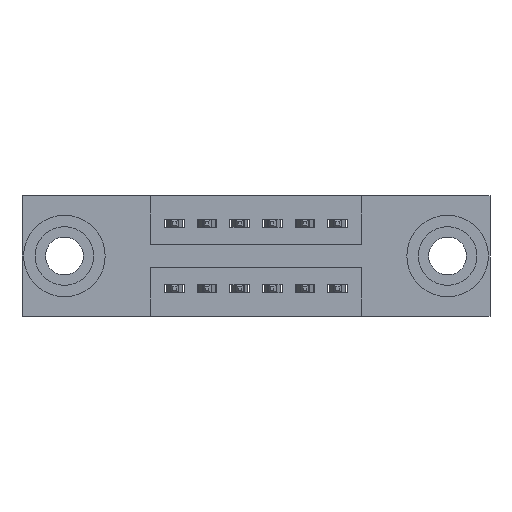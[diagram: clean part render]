
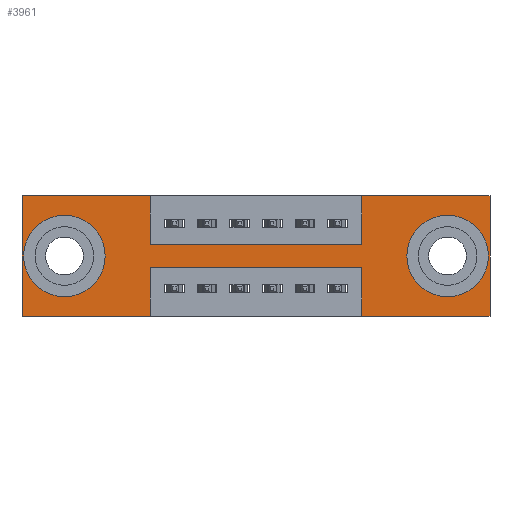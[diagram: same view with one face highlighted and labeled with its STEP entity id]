
A CAD part, front view. The second image highlights one B-rep face of the part: STEP entity #3961.
In plain terms, the highlighted planar face has unit normal (0, -1, 0).
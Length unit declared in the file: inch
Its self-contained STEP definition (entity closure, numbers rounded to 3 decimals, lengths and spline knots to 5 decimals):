
#34 = DIRECTION ( 'NONE',  ( 0., 0., -1. ) ) ;
#42 = VERTEX_POINT ( 'NONE', #1197 ) ;
#92 = CARTESIAN_POINT ( 'NONE',  ( 0., 0., -0.37 ) ) ;
#171 = DIRECTION ( 'NONE',  ( 1., 0., 0. ) ) ;
#291 = ORIENTED_EDGE ( 'NONE', *, *, #3632, .F. ) ;
#335 = AXIS2_PLACEMENT_3D ( 'NONE', #6196, #7779, #588 ) ;
#345 = CARTESIAN_POINT ( 'NONE',  ( 0.13, 0., -0.185 ) ) ;
#395 = ORIENTED_EDGE ( 'NONE', *, *, #940, .F. ) ;
#414 = VERTEX_POINT ( 'NONE', #714 ) ;
#434 = DIRECTION ( 'NONE',  ( 0., -1., 0. ) ) ;
#467 = CARTESIAN_POINT ( 'NONE',  ( 0., 0., 0. ) ) ;
#563 = EDGE_CURVE ( 'NONE', #6876, #4122, #4828, .T. ) ;
#571 = CARTESIAN_POINT ( 'NONE',  ( 1.0425, 0., 0. ) ) ;
#588 = DIRECTION ( 'NONE',  ( 0., 0., -1. ) ) ;
#666 = ORIENTED_EDGE ( 'NONE', *, *, #8290, .F. ) ;
#674 = VECTOR ( 'NONE', #724, 39.37008 ) ;
#714 = CARTESIAN_POINT ( 'NONE',  ( 0.3925, 0., -0.22 ) ) ;
#724 = DIRECTION ( 'NONE',  ( 1., 0., 0. ) ) ;
#737 = EDGE_CURVE ( 'NONE', #7230, #2003, #8035, .T. ) ;
#739 = CIRCLE ( 'NONE', #6644, 0.078 ) ;
#795 = ORIENTED_EDGE ( 'NONE', *, *, #1327, .F. ) ;
#940 = EDGE_CURVE ( 'NONE', #2744, #7206, #5294, .T. ) ;
#1187 = VECTOR ( 'NONE', #8932, 39.37008 ) ;
#1197 = CARTESIAN_POINT ( 'NONE',  ( 0.3925, 0., -0.15 ) ) ;
#1201 = VECTOR ( 'NONE', #8632, 39.37008 ) ;
#1287 = EDGE_CURVE ( 'NONE', #6546, #9096, #7022, .T. ) ;
#1300 = DIRECTION ( 'NONE',  ( 1., 0., 0. ) ) ;
#1327 = EDGE_CURVE ( 'NONE', #4214, #7230, #3807, .T. ) ;
#1444 = EDGE_CURVE ( 'NONE', #6327, #7670, #5656, .T. ) ;
#1595 = ORIENTED_EDGE ( 'NONE', *, *, #1444, .F. ) ;
#1898 = EDGE_CURVE ( 'NONE', #9096, #6546, #739, .T. ) ;
#1931 = LINE ( 'NONE', #2389, #1201 ) ;
#2003 = VERTEX_POINT ( 'NONE', #5486 ) ;
#2044 = CARTESIAN_POINT ( 'NONE',  ( 1.0425, 0., 0. ) ) ;
#2093 = EDGE_CURVE ( 'NONE', #8077, #414, #1931, .T. ) ;
#2120 = LINE ( 'NONE', #4509, #7315 ) ;
#2130 = VECTOR ( 'NONE', #1300, 39.37008 ) ;
#2210 = ORIENTED_EDGE ( 'NONE', *, *, #3200, .T. ) ;
#2382 = LINE ( 'NONE', #9507, #8199 ) ;
#2389 = CARTESIAN_POINT ( 'NONE',  ( 0.3925, 0., -0.22 ) ) ;
#2440 = EDGE_LOOP ( 'NONE', ( #5315, #8409 ) ) ;
#2575 = VECTOR ( 'NONE', #8770, 39.37008 ) ;
#2744 = VERTEX_POINT ( 'NONE', #4834 ) ;
#2754 = EDGE_LOOP ( 'NONE', ( #7285, #3383, #3017, #5675, #795, #291, #395, #4538, #8168, #666, #6199, #1595 ) ) ;
#2786 = PLANE ( 'NONE',  #6846 ) ;
#2809 = VECTOR ( 'NONE', #9680, 39.37008 ) ;
#2816 = VECTOR ( 'NONE', #171, 39.37008 ) ;
#2968 = CARTESIAN_POINT ( 'NONE',  ( 1.435, 0., -0.37 ) ) ;
#3017 = ORIENTED_EDGE ( 'NONE', *, *, #5569, .F. ) ;
#3023 = EDGE_CURVE ( 'NONE', #414, #6327, #8112, .T. ) ;
#3105 = DIRECTION ( 'NONE',  ( 0., 1., 0. ) ) ;
#3200 = EDGE_CURVE ( 'NONE', #4122, #6876, #6123, .T. ) ;
#3363 = CARTESIAN_POINT ( 'NONE',  ( 0.3925, 0., -0.37 ) ) ;
#3383 = ORIENTED_EDGE ( 'NONE', *, *, #2093, .F. ) ;
#3570 = DIRECTION ( 'NONE',  ( 0., 0., 1. ) ) ;
#3632 = EDGE_CURVE ( 'NONE', #7206, #4214, #7456, .T. ) ;
#3633 = FACE_BOUND ( 'NONE', #3957, .T. ) ;
#3665 = CARTESIAN_POINT ( 'NONE',  ( 1.0425, 0., -0.37 ) ) ;
#3807 = LINE ( 'NONE', #7151, #2575 ) ;
#3957 = EDGE_LOOP ( 'NONE', ( #7525, #2210 ) ) ;
#3961 = ADVANCED_FACE ( 'NONE', ( #3633, #7321, #5119 ), #2786, .T. ) ;
#4122 = VERTEX_POINT ( 'NONE', #8768 ) ;
#4139 = DIRECTION ( 'NONE',  ( 0., 1., 0. ) ) ;
#4182 = CARTESIAN_POINT ( 'NONE',  ( 0., 0., -0.37 ) ) ;
#4214 = VERTEX_POINT ( 'NONE', #7211 ) ;
#4333 = VECTOR ( 'NONE', #8064, 39.37008 ) ;
#4413 = VECTOR ( 'NONE', #5280, 39.37008 ) ;
#4509 = CARTESIAN_POINT ( 'NONE',  ( 0.3925, 0., 0. ) ) ;
#4538 = ORIENTED_EDGE ( 'NONE', *, *, #4627, .F. ) ;
#4627 = EDGE_CURVE ( 'NONE', #42, #2744, #4930, .T. ) ;
#4649 = AXIS2_PLACEMENT_3D ( 'NONE', #5413, #4139, #34 ) ;
#4743 = DIRECTION ( 'NONE',  ( 0., 0., 1. ) ) ;
#4828 = CIRCLE ( 'NONE', #4649, 0.078 ) ;
#4834 = CARTESIAN_POINT ( 'NONE',  ( 1.0425, 0., -0.15 ) ) ;
#4930 = LINE ( 'NONE', #8041, #2816 ) ;
#5119 = FACE_OUTER_BOUND ( 'NONE', #2754, .T. ) ;
#5280 = DIRECTION ( 'NONE',  ( 0., 0., 1. ) ) ;
#5294 = LINE ( 'NONE', #2044, #6050 ) ;
#5315 = ORIENTED_EDGE ( 'NONE', *, *, #1287, .T. ) ;
#5323 = CARTESIAN_POINT ( 'NONE',  ( 0.13, 0., -0.107 ) ) ;
#5381 = CARTESIAN_POINT ( 'NONE',  ( 0., 0., 0. ) ) ;
#5413 = CARTESIAN_POINT ( 'NONE',  ( 1.305, 0., -0.185 ) ) ;
#5486 = CARTESIAN_POINT ( 'NONE',  ( 1.0425, 0., -0.37 ) ) ;
#5569 = EDGE_CURVE ( 'NONE', #2003, #8077, #9389, .T. ) ;
#5656 = LINE ( 'NONE', #92, #2809 ) ;
#5675 = ORIENTED_EDGE ( 'NONE', *, *, #737, .F. ) ;
#5862 = CARTESIAN_POINT ( 'NONE',  ( 0., 0., 0. ) ) ;
#5942 = DIRECTION ( 'NONE',  ( 0., 0., -1. ) ) ;
#6004 = DIRECTION ( 'NONE',  ( 0., 0., 1. ) ) ;
#6050 = VECTOR ( 'NONE', #6004, 39.37008 ) ;
#6123 = CIRCLE ( 'NONE', #335, 0.078 ) ;
#6196 = CARTESIAN_POINT ( 'NONE',  ( 1.305, 0., -0.185 ) ) ;
#6199 = ORIENTED_EDGE ( 'NONE', *, *, #8209, .F. ) ;
#6327 = VERTEX_POINT ( 'NONE', #8201 ) ;
#6340 = DIRECTION ( 'NONE',  ( 0., 0., 1. ) ) ;
#6546 = VERTEX_POINT ( 'NONE', #5323 ) ;
#6644 = AXIS2_PLACEMENT_3D ( 'NONE', #345, #8214, #3570 ) ;
#6846 = AXIS2_PLACEMENT_3D ( 'NONE', #7477, #434, #5942 ) ;
#6876 = VERTEX_POINT ( 'NONE', #7861 ) ;
#6920 = CARTESIAN_POINT ( 'NONE',  ( 1.0425, 0., -0.22 ) ) ;
#7022 = CIRCLE ( 'NONE', #9207, 0.078 ) ;
#7151 = CARTESIAN_POINT ( 'NONE',  ( 1.435, 0., 0. ) ) ;
#7206 = VERTEX_POINT ( 'NONE', #571 ) ;
#7211 = CARTESIAN_POINT ( 'NONE',  ( 1.435, 0., 0. ) ) ;
#7230 = VERTEX_POINT ( 'NONE', #2968 ) ;
#7285 = ORIENTED_EDGE ( 'NONE', *, *, #3023, .F. ) ;
#7295 = LINE ( 'NONE', #5381, #674 ) ;
#7315 = VECTOR ( 'NONE', #8509, 39.37008 ) ;
#7321 = FACE_BOUND ( 'NONE', #2440, .T. ) ;
#7450 = CARTESIAN_POINT ( 'NONE',  ( 0., 0., -0.37 ) ) ;
#7456 = LINE ( 'NONE', #467, #2130 ) ;
#7477 = CARTESIAN_POINT ( 'NONE',  ( 0., 0., -0.37 ) ) ;
#7525 = ORIENTED_EDGE ( 'NONE', *, *, #563, .T. ) ;
#7670 = VERTEX_POINT ( 'NONE', #7450 ) ;
#7692 = EDGE_CURVE ( 'NONE', #8087, #42, #2120, .T. ) ;
#7779 = DIRECTION ( 'NONE',  ( 0., 1., 0. ) ) ;
#7861 = CARTESIAN_POINT ( 'NONE',  ( 1.305, 0., -0.107 ) ) ;
#8035 = LINE ( 'NONE', #4182, #4333 ) ;
#8041 = CARTESIAN_POINT ( 'NONE',  ( 0.3925, 0., -0.15 ) ) ;
#8064 = DIRECTION ( 'NONE',  ( -1., 0., 0. ) ) ;
#8077 = VERTEX_POINT ( 'NONE', #6920 ) ;
#8087 = VERTEX_POINT ( 'NONE', #8548 ) ;
#8112 = LINE ( 'NONE', #3363, #1187 ) ;
#8168 = ORIENTED_EDGE ( 'NONE', *, *, #7692, .F. ) ;
#8199 = VECTOR ( 'NONE', #4743, 39.37008 ) ;
#8201 = CARTESIAN_POINT ( 'NONE',  ( 0.3925, 0., -0.37 ) ) ;
#8209 = EDGE_CURVE ( 'NONE', #7670, #9990, #2382, .T. ) ;
#8214 = DIRECTION ( 'NONE',  ( 0., 1., 0. ) ) ;
#8290 = EDGE_CURVE ( 'NONE', #9990, #8087, #7295, .T. ) ;
#8409 = ORIENTED_EDGE ( 'NONE', *, *, #1898, .T. ) ;
#8509 = DIRECTION ( 'NONE',  ( 0., 0., -1. ) ) ;
#8548 = CARTESIAN_POINT ( 'NONE',  ( 0.3925, 0., 0. ) ) ;
#8632 = DIRECTION ( 'NONE',  ( -1., 0., 0. ) ) ;
#8674 = CARTESIAN_POINT ( 'NONE',  ( 0.13, 0., -0.185 ) ) ;
#8768 = CARTESIAN_POINT ( 'NONE',  ( 1.305, 0., -0.263 ) ) ;
#8770 = DIRECTION ( 'NONE',  ( 0., 0., -1. ) ) ;
#8932 = DIRECTION ( 'NONE',  ( 0., 0., -1. ) ) ;
#9096 = VERTEX_POINT ( 'NONE', #9243 ) ;
#9207 = AXIS2_PLACEMENT_3D ( 'NONE', #8674, #3105, #6340 ) ;
#9243 = CARTESIAN_POINT ( 'NONE',  ( 0.13, 0., -0.263 ) ) ;
#9389 = LINE ( 'NONE', #3665, #4413 ) ;
#9507 = CARTESIAN_POINT ( 'NONE',  ( 0., 0., 0. ) ) ;
#9680 = DIRECTION ( 'NONE',  ( -1., 0., 0. ) ) ;
#9990 = VERTEX_POINT ( 'NONE', #5862 ) ;
